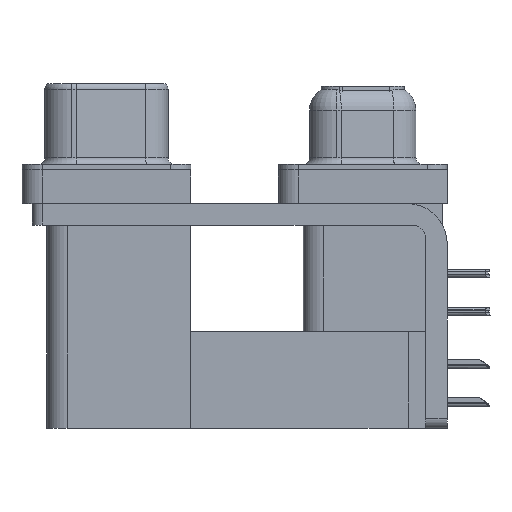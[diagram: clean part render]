
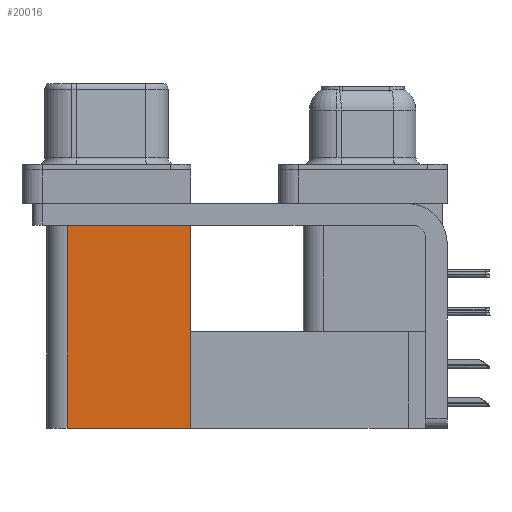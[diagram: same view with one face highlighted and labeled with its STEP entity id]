
A CAD part, left-side view. The second image highlights one B-rep face of the part: STEP entity #20016.
In plain terms, the highlighted planar face has unit normal (-1, 0, 0).
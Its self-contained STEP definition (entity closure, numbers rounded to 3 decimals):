
#101 = EDGE_CURVE ( 'NONE', #43351, #12060, #17321, .T. ) ;
#220 = VECTOR ( 'NONE', #28721, 1000. ) ;
#750 = CARTESIAN_POINT ( 'NONE',  ( 3.7, 12.775, -19.2 ) ) ;
#2284 = LINE ( 'NONE', #26389, #16256 ) ;
#3420 = DIRECTION ( 'NONE',  ( 0., 1., 0. ) ) ;
#3688 = CARTESIAN_POINT ( 'NONE',  ( 3.7, 12.775, -19.2 ) ) ;
#6093 = CARTESIAN_POINT ( 'NONE',  ( 3.7, 12.775, -19.2 ) ) ;
#10838 = DIRECTION ( 'NONE',  ( 1., 0., 0. ) ) ;
#12060 = VERTEX_POINT ( 'NONE', #51738 ) ;
#12319 = DIRECTION ( 'NONE',  ( 0., 0., 1. ) ) ;
#12526 = EDGE_CURVE ( 'NONE', #51026, #43351, #2284, .T. ) ;
#14323 = VECTOR ( 'NONE', #12319, 1000. ) ;
#16256 = VECTOR ( 'NONE', #26642, 1000. ) ;
#16425 = EDGE_CURVE ( 'NONE', #44176, #12060, #28233, .T. ) ;
#17321 = LINE ( 'NONE', #32964, #220 ) ;
#20016 = ADVANCED_FACE ( 'NONE', ( #46955 ), #26745, .F. ) ;
#20049 = ORIENTED_EDGE ( 'NONE', *, *, #101, .T. ) ;
#20276 = CARTESIAN_POINT ( 'NONE',  ( 3.7, 21.975, -19.2 ) ) ;
#21140 = LINE ( 'NONE', #750, #47610 ) ;
#24643 = ORIENTED_EDGE ( 'NONE', *, *, #12526, .T. ) ;
#26389 = CARTESIAN_POINT ( 'NONE',  ( 3.7, 12.775, -19.2 ) ) ;
#26642 = DIRECTION ( 'NONE',  ( 0., 0., 1. ) ) ;
#26745 = PLANE ( 'NONE',  #49030 ) ;
#28233 = LINE ( 'NONE', #20276, #14323 ) ;
#28721 = DIRECTION ( 'NONE',  ( 0., 1., 0. ) ) ;
#32322 = ORIENTED_EDGE ( 'NONE', *, *, #51424, .F. ) ;
#32964 = CARTESIAN_POINT ( 'NONE',  ( 3.7, 12.775, -2.5 ) ) ;
#33345 = DIRECTION ( 'NONE',  ( 0., 1., 0. ) ) ;
#37369 = CARTESIAN_POINT ( 'NONE',  ( 3.7, 12.775, -2.5 ) ) ;
#39242 = CARTESIAN_POINT ( 'NONE',  ( 3.7, 21.975, -19.2 ) ) ;
#43351 = VERTEX_POINT ( 'NONE', #37369 ) ;
#44176 = VERTEX_POINT ( 'NONE', #39242 ) ;
#46159 = EDGE_LOOP ( 'NONE', ( #20049, #46255, #32322, #24643 ) ) ;
#46255 = ORIENTED_EDGE ( 'NONE', *, *, #16425, .F. ) ;
#46955 = FACE_OUTER_BOUND ( 'NONE', #46159, .T. ) ;
#47610 = VECTOR ( 'NONE', #33345, 1000. ) ;
#49030 = AXIS2_PLACEMENT_3D ( 'NONE', #3688, #10838, #3420 ) ;
#51026 = VERTEX_POINT ( 'NONE', #6093 ) ;
#51424 = EDGE_CURVE ( 'NONE', #51026, #44176, #21140, .T. ) ;
#51738 = CARTESIAN_POINT ( 'NONE',  ( 3.7, 21.975, -2.5 ) ) ;
